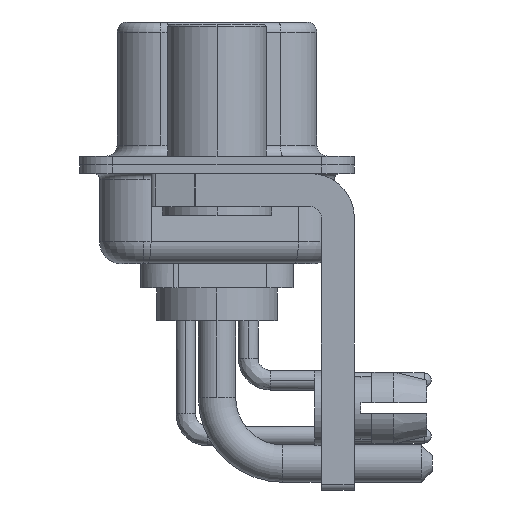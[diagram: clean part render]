
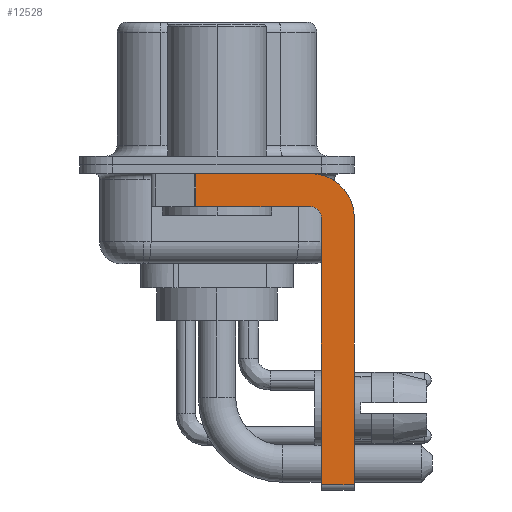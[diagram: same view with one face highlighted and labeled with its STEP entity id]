
A CAD part, left-side view. The second image highlights one B-rep face of the part: STEP entity #12528.
In plain terms, the highlighted planar face has unit normal (-1, 0, 0).
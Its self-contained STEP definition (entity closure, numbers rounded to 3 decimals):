
#613 = LINE ( 'NONE', #9954, #14333 ) ;
#777 = ORIENTED_EDGE ( 'NONE', *, *, #26413, .F. ) ;
#2130 = VECTOR ( 'NONE', #23144, 1000. ) ;
#2816 = CARTESIAN_POINT ( 'NONE',  ( -2.9, -6.25, -2.4 ) ) ;
#3431 = CARTESIAN_POINT ( 'NONE',  ( -2.9, -6.25, -14.55 ) ) ;
#3657 = CARTESIAN_POINT ( 'NONE',  ( -2.9, -4.25, -2.4 ) ) ;
#3671 = ORIENTED_EDGE ( 'NONE', *, *, #15475, .F. ) ;
#3687 = LINE ( 'NONE', #10434, #5067 ) ;
#3696 = CARTESIAN_POINT ( 'NONE',  ( -2.9, -6.25, -2.4 ) ) ;
#3746 = CARTESIAN_POINT ( 'NONE',  ( -2.9, -4.25, -1.9 ) ) ;
#3926 = VERTEX_POINT ( 'NONE', #3746 ) ;
#4774 = ORIENTED_EDGE ( 'NONE', *, *, #19419, .F. ) ;
#5067 = VECTOR ( 'NONE', #26692, 1000. ) ;
#5357 = DIRECTION ( 'NONE',  ( 0., -1., 0. ) ) ;
#5383 = ORIENTED_EDGE ( 'NONE', *, *, #15846, .F. ) ;
#5457 = ORIENTED_EDGE ( 'NONE', *, *, #16733, .F. ) ;
#5502 = CARTESIAN_POINT ( 'NONE',  ( -2.9, -4.75, -14.55 ) ) ;
#5674 = ORIENTED_EDGE ( 'NONE', *, *, #22425, .T. ) ;
#5826 = AXIS2_PLACEMENT_3D ( 'NONE', #11513, #29937, #11064 ) ;
#7319 = FACE_OUTER_BOUND ( 'NONE', #24923, .T. ) ;
#7519 = VECTOR ( 'NONE', #13029, 1000. ) ;
#7731 = LINE ( 'NONE', #8183, #22282 ) ;
#8022 = CIRCLE ( 'NONE', #11476, 0.5 ) ;
#8183 = CARTESIAN_POINT ( 'NONE',  ( -2.9, -4.25, -1.9 ) ) ;
#8897 = CARTESIAN_POINT ( 'NONE',  ( -2.9, 0.978, -1.9 ) ) ;
#9743 = CARTESIAN_POINT ( 'NONE',  ( -2.9, -4.75, -2.4 ) ) ;
#9770 = DIRECTION ( 'NONE',  ( 0., 0., -1. ) ) ;
#9954 = CARTESIAN_POINT ( 'NONE',  ( -2.9, -4.25, -14.55 ) ) ;
#10434 = CARTESIAN_POINT ( 'NONE',  ( -2.9, 3., -0.4 ) ) ;
#10484 = DIRECTION ( 'NONE',  ( 0., 1., 0. ) ) ;
#10928 = VERTEX_POINT ( 'NONE', #17856 ) ;
#11064 = DIRECTION ( 'NONE',  ( 0., 0., -1. ) ) ;
#11476 = AXIS2_PLACEMENT_3D ( 'NONE', #3657, #26662, #17168 ) ;
#11513 = CARTESIAN_POINT ( 'NONE',  ( -2.9, -4.25, -2.4 ) ) ;
#12292 = DIRECTION ( 'NONE',  ( 0., 0., 1. ) ) ;
#12528 = ADVANCED_FACE ( 'NONE', ( #7319 ), #29072, .F. ) ;
#13029 = DIRECTION ( 'NONE',  ( 0., 0., -1. ) ) ;
#13242 = VERTEX_POINT ( 'NONE', #3431 ) ;
#13243 = AXIS2_PLACEMENT_3D ( 'NONE', #28933, #17276, #9770 ) ;
#14333 = VECTOR ( 'NONE', #5357, 1000. ) ;
#15092 = VERTEX_POINT ( 'NONE', #2816 ) ;
#15475 = EDGE_CURVE ( 'NONE', #15092, #13242, #24706, .T. ) ;
#15846 = EDGE_CURVE ( 'NONE', #16532, #3926, #8022, .T. ) ;
#16532 = VERTEX_POINT ( 'NONE', #9743 ) ;
#16613 = CARTESIAN_POINT ( 'NONE',  ( -2.9, 0.978, -0.4 ) ) ;
#16733 = EDGE_CURVE ( 'NONE', #3926, #19633, #7731, .T. ) ;
#16906 = LINE ( 'NONE', #28406, #20377 ) ;
#17168 = DIRECTION ( 'NONE',  ( 0., 0., 1. ) ) ;
#17276 = DIRECTION ( 'NONE',  ( 1., 0., 0. ) ) ;
#17856 = CARTESIAN_POINT ( 'NONE',  ( -2.9, -4.25, -0.4 ) ) ;
#18042 = ORIENTED_EDGE ( 'NONE', *, *, #21100, .T. ) ;
#19419 = EDGE_CURVE ( 'NONE', #27794, #10928, #3687, .T. ) ;
#19633 = VERTEX_POINT ( 'NONE', #8897 ) ;
#20377 = VECTOR ( 'NONE', #12292, 1000. ) ;
#20540 = LINE ( 'NONE', #25312, #2130 ) ;
#21020 = CIRCLE ( 'NONE', #5826, 2. ) ;
#21034 = VERTEX_POINT ( 'NONE', #5502 ) ;
#21100 = EDGE_CURVE ( 'NONE', #21034, #13242, #613, .T. ) ;
#22282 = VECTOR ( 'NONE', #10484, 1000. ) ;
#22425 = EDGE_CURVE ( 'NONE', #27794, #19633, #20540, .T. ) ;
#23144 = DIRECTION ( 'NONE',  ( 0., 0., -1. ) ) ;
#24706 = LINE ( 'NONE', #3696, #7519 ) ;
#24923 = EDGE_LOOP ( 'NONE', ( #4774, #5674, #5457, #5383, #777, #18042, #3671, #25839 ) ) ;
#25312 = CARTESIAN_POINT ( 'NONE',  ( -2.9, 0.978, -1.9 ) ) ;
#25839 = ORIENTED_EDGE ( 'NONE', *, *, #29276, .F. ) ;
#26413 = EDGE_CURVE ( 'NONE', #21034, #16532, #16906, .T. ) ;
#26662 = DIRECTION ( 'NONE',  ( -1., 0., 0. ) ) ;
#26692 = DIRECTION ( 'NONE',  ( 0., -1., 0. ) ) ;
#27794 = VERTEX_POINT ( 'NONE', #16613 ) ;
#28406 = CARTESIAN_POINT ( 'NONE',  ( -2.9, -4.75, -14.8 ) ) ;
#28933 = CARTESIAN_POINT ( 'NONE',  ( -2.9, -4.25, -2.4 ) ) ;
#29072 = PLANE ( 'NONE',  #13243 ) ;
#29276 = EDGE_CURVE ( 'NONE', #10928, #15092, #21020, .T. ) ;
#29937 = DIRECTION ( 'NONE',  ( 1., 0., 0. ) ) ;
